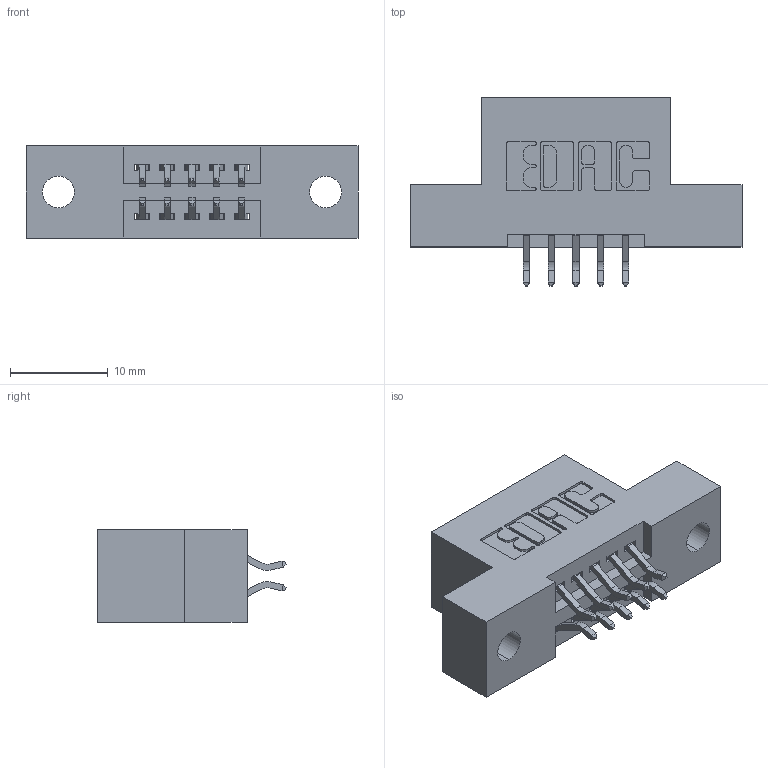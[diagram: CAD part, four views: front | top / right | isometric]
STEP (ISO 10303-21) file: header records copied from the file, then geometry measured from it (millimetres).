
FILE_DESCRIPTION (( 'STEP AP203' ), '1' );
FILE_NAME ('345-010-556-202.STEP', '2018-08-17T21:34:10', ( '' ), ( '' ), 'SwSTEP 2.0', 'SolidWorks 2016', '' );
FILE_SCHEMA (( 'CONFIG_CONTROL_DESIGN' ));
Length unit declared in the file: inch
Products named in the file (3): 345 Part_Flush Mounting Lugs - 0.128 Dia; 345-292-001_556 Tail; 345-010-556-202
Assembly tree (11 placements, depth 2):
  345-010-556-202
    345 Part_Flush Mounting Lugs - 0.128 Dia
    345-292-001_556 Tail  x10
Bounding box: 33.91 x 19.24 x 9.4 mm (x, y, z)
Volume: 2913.4 mm3; surface area: 3308.4 mm2
Topology: 11 solids, 11 shells, 686 faces, 2011 edges, 1326 vertices
Faces by surface type: plane 450, cylinder 236
Entity records: 9127 total; most frequent: CARTESIAN_POINT 1580, ORIENTED_EDGE 1502, DIRECTION 1427, EDGE_CURVE 751, VECTOR 591, LINE 591, VERTEX_POINT 498, AXIS2_PLACEMENT_3D 418
